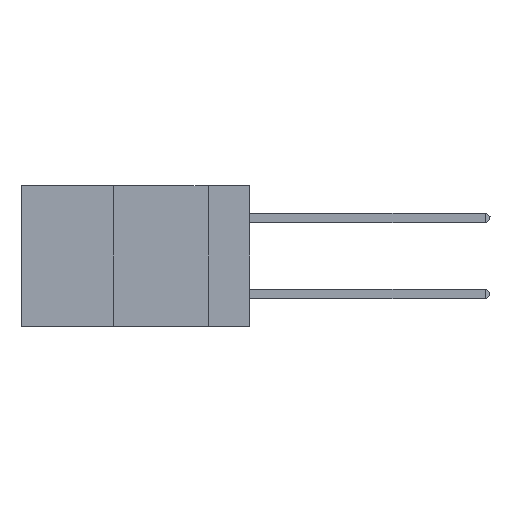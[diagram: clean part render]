
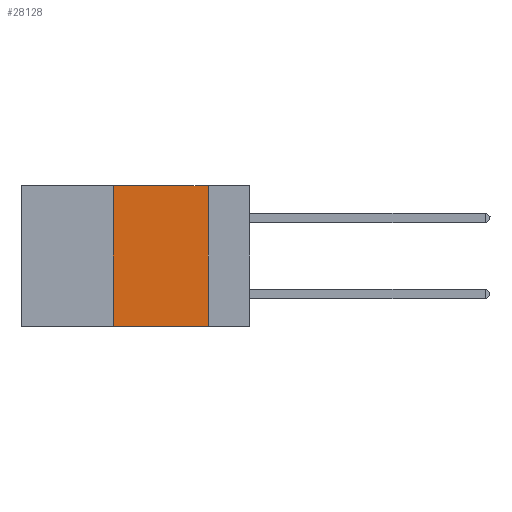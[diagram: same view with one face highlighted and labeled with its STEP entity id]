
A CAD part, left-side view. The second image highlights one B-rep face of the part: STEP entity #28128.
In plain terms, the highlighted planar face has unit normal (-1, 0, 0).
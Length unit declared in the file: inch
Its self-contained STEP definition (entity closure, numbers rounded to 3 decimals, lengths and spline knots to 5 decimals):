
#486 = ORIENTED_EDGE ( 'NONE', *, *, #6619, .F. ) ;
#1991 = FACE_OUTER_BOUND ( 'NONE', #27757, .T. ) ;
#4486 = EDGE_CURVE ( 'NONE', #40543, #39220, #35726, .T. ) ;
#5739 = DIRECTION ( 'NONE',  ( 1., 0., 0. ) ) ;
#6189 = EDGE_CURVE ( 'NONE', #39220, #30033, #8937, .T. ) ;
#6619 = EDGE_CURVE ( 'NONE', #23556, #40543, #43489, .T. ) ;
#8245 = DIRECTION ( 'NONE',  ( 0., 0., -1. ) ) ;
#8937 = LINE ( 'NONE', #36109, #40703 ) ;
#9229 = CARTESIAN_POINT ( 'NONE',  ( 0., 0.6, 0. ) ) ;
#11700 = CARTESIAN_POINT ( 'NONE',  ( 0., 0.36, 0. ) ) ;
#13704 = DIRECTION ( 'NONE',  ( 0., -1., 0. ) ) ;
#14618 = DIRECTION ( 'NONE',  ( 0., -1., 0. ) ) ;
#16971 = AXIS2_PLACEMENT_3D ( 'NONE', #9229, #5739, #40560 ) ;
#20106 = PLANE ( 'NONE',  #16971 ) ;
#21338 = CARTESIAN_POINT ( 'NONE',  ( 0., 0.6, 0. ) ) ;
#23556 = VERTEX_POINT ( 'NONE', #27213 ) ;
#24711 = VECTOR ( 'NONE', #13704, 39.37008 ) ;
#27213 = CARTESIAN_POINT ( 'NONE',  ( 0., 0.36, -0.37 ) ) ;
#27415 = CARTESIAN_POINT ( 'NONE',  ( 0., 0.6, -0.37 ) ) ;
#27757 = EDGE_LOOP ( 'NONE', ( #37603, #42944, #486, #29121 ) ) ;
#28084 = LINE ( 'NONE', #27415, #24711 ) ;
#28128 = ADVANCED_FACE ( 'NONE', ( #1991 ), #20106, .F. ) ;
#28337 = CARTESIAN_POINT ( 'NONE',  ( 0., 0.11, 0. ) ) ;
#29121 = ORIENTED_EDGE ( 'NONE', *, *, #34809, .T. ) ;
#30033 = VERTEX_POINT ( 'NONE', #35126 ) ;
#34809 = EDGE_CURVE ( 'NONE', #23556, #30033, #28084, .T. ) ;
#35126 = CARTESIAN_POINT ( 'NONE',  ( 0., 0.11, -0.37 ) ) ;
#35726 = LINE ( 'NONE', #21338, #45073 ) ;
#36109 = CARTESIAN_POINT ( 'NONE',  ( 0., 0.11, 0. ) ) ;
#37603 = ORIENTED_EDGE ( 'NONE', *, *, #6189, .F. ) ;
#39220 = VERTEX_POINT ( 'NONE', #28337 ) ;
#39540 = DIRECTION ( 'NONE',  ( 0., 0., 1. ) ) ;
#39679 = VECTOR ( 'NONE', #39540, 39.37008 ) ;
#40543 = VERTEX_POINT ( 'NONE', #45306 ) ;
#40560 = DIRECTION ( 'NONE',  ( 0., 0., -1. ) ) ;
#40703 = VECTOR ( 'NONE', #8245, 39.37008 ) ;
#42944 = ORIENTED_EDGE ( 'NONE', *, *, #4486, .F. ) ;
#43489 = LINE ( 'NONE', #11700, #39679 ) ;
#45073 = VECTOR ( 'NONE', #14618, 39.37008 ) ;
#45306 = CARTESIAN_POINT ( 'NONE',  ( 0., 0.36, 0. ) ) ;
